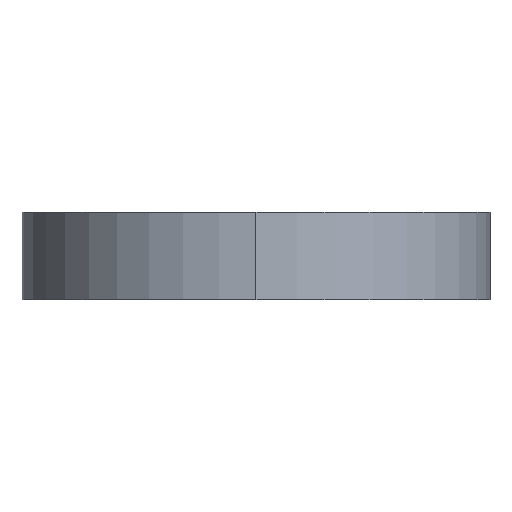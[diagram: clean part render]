
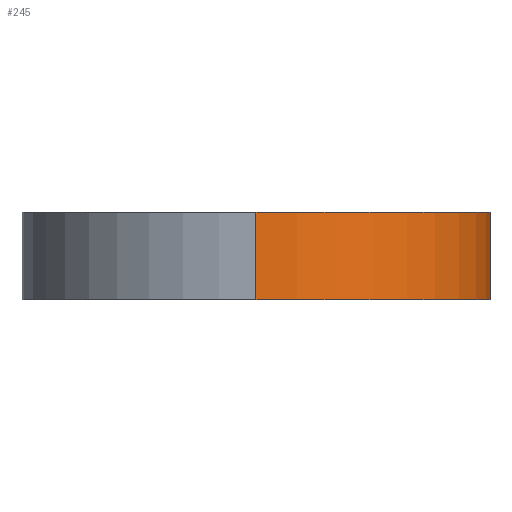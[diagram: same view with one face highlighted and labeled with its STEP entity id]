
A CAD part, front view. The second image highlights one B-rep face of the part: STEP entity #245.
In plain terms, the highlighted cylindrical face has radius 27 mm (diameter 54 mm), a partial arc.
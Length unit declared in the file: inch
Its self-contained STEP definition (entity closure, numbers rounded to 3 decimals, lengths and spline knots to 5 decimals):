
#6 = DIRECTION ( 'NONE',  ( 0., 0., -1. ) ) ;
#62 = AXIS2_PLACEMENT_3D ( 'NONE', #313, #6, #166 ) ;
#80 = CARTESIAN_POINT ( 'NONE',  ( 0.64854, -1.31854, 0.12481 ) ) ;
#88 = AXIS2_PLACEMENT_3D ( 'NONE', #480, #602, #158 ) ;
#111 = EDGE_CURVE ( 'NONE', #612, #165, #547, .T. ) ;
#138 = AXIS2_PLACEMENT_3D ( 'NONE', #652, #160, #610 ) ;
#158 = DIRECTION ( 'NONE',  ( 0., 1., 0. ) ) ;
#160 = DIRECTION ( 'NONE',  ( 0., 0., 1. ) ) ;
#165 = VERTEX_POINT ( 'NONE', #212 ) ;
#166 = DIRECTION ( 'NONE',  ( 0., 1., 0. ) ) ;
#212 = CARTESIAN_POINT ( 'NONE',  ( -0.40774, -2.38151, 0.51851 ) ) ;
#228 = LINE ( 'NONE', #666, #394 ) ;
#245 = ADVANCED_FACE ( 'NONE', ( #268 ), #404, .T. ) ;
#252 = EDGE_CURVE ( 'NONE', #520, #489, #714, .T. ) ;
#268 = FACE_OUTER_BOUND ( 'NONE', #370, .T. ) ;
#271 = DIRECTION ( 'NONE',  ( 0., 0., 1. ) ) ;
#313 = CARTESIAN_POINT ( 'NONE',  ( -0.41445, -1.31854, 0.12481 ) ) ;
#332 = ORIENTED_EDGE ( 'NONE', *, *, #111, .T. ) ;
#340 = EDGE_CURVE ( 'NONE', #520, #612, #559, .T. ) ;
#343 = CARTESIAN_POINT ( 'NONE',  ( 0.64854, -1.31854, 0.51851 ) ) ;
#367 = DIRECTION ( 'NONE',  ( 0., 0., 1. ) ) ;
#370 = EDGE_LOOP ( 'NONE', ( #332, #644, #433, #518 ) ) ;
#375 = CARTESIAN_POINT ( 'NONE',  ( 0.64854, -1.31854, 0.12481 ) ) ;
#394 = VECTOR ( 'NONE', #271, 39.37008 ) ;
#404 = CYLINDRICAL_SURFACE ( 'NONE', #138, 1.06299 ) ;
#433 = ORIENTED_EDGE ( 'NONE', *, *, #252, .F. ) ;
#466 = EDGE_CURVE ( 'NONE', #489, #165, #228, .T. ) ;
#480 = CARTESIAN_POINT ( 'NONE',  ( -0.41445, -1.31854, 0.51851 ) ) ;
#489 = VERTEX_POINT ( 'NONE', #658 ) ;
#518 = ORIENTED_EDGE ( 'NONE', *, *, #340, .T. ) ;
#520 = VERTEX_POINT ( 'NONE', #80 ) ;
#537 = VECTOR ( 'NONE', #367, 39.37008 ) ;
#547 = CIRCLE ( 'NONE', #88, 1.06299 ) ;
#559 = LINE ( 'NONE', #375, #537 ) ;
#602 = DIRECTION ( 'NONE',  ( 0., 0., -1. ) ) ;
#610 = DIRECTION ( 'NONE',  ( 0., -1., 0. ) ) ;
#612 = VERTEX_POINT ( 'NONE', #343 ) ;
#644 = ORIENTED_EDGE ( 'NONE', *, *, #466, .F. ) ;
#652 = CARTESIAN_POINT ( 'NONE',  ( -0.41445, -1.31854, 0.12481 ) ) ;
#658 = CARTESIAN_POINT ( 'NONE',  ( -0.40774, -2.38151, 0.12481 ) ) ;
#666 = CARTESIAN_POINT ( 'NONE',  ( -0.40774, -2.38151, 0.12481 ) ) ;
#714 = CIRCLE ( 'NONE', #62, 1.06299 ) ;
